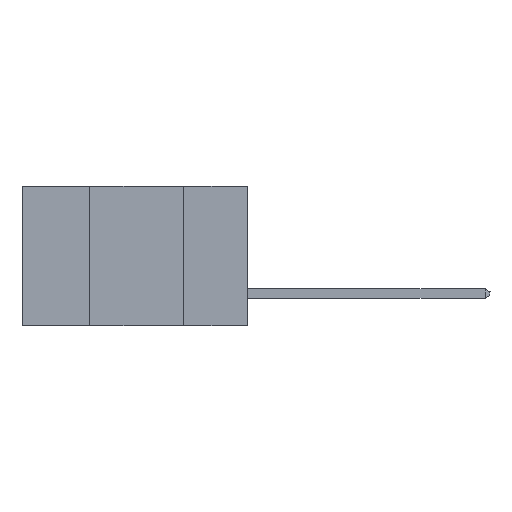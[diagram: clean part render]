
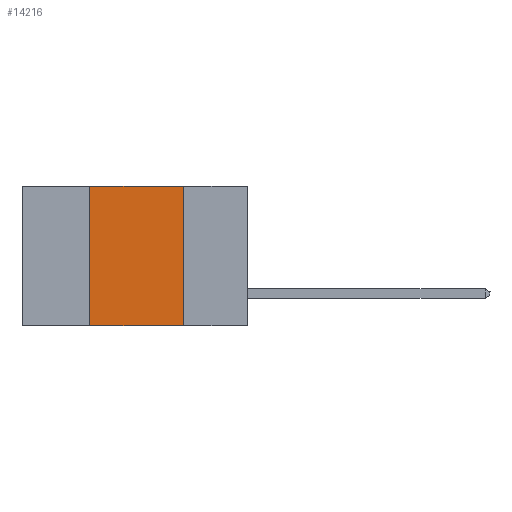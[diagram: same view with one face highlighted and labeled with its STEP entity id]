
A CAD part, left-side view. The second image highlights one B-rep face of the part: STEP entity #14216.
In plain terms, the highlighted planar face has unit normal (-1, 0, 0).
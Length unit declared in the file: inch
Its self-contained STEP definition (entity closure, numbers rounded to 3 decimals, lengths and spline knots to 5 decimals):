
#107 = CARTESIAN_POINT ( 'NONE',  ( 0., 0.17, -0.37 ) ) ;
#370 = VECTOR ( 'NONE', #12506, 39.37008 ) ;
#591 = LINE ( 'NONE', #22210, #370 ) ;
#2388 = LINE ( 'NONE', #23874, #9001 ) ;
#3437 = DIRECTION ( 'NONE',  ( 1., 0., 0. ) ) ;
#3666 = ORIENTED_EDGE ( 'NONE', *, *, #16889, .F. ) ;
#3943 = LINE ( 'NONE', #25311, #14089 ) ;
#4243 = CARTESIAN_POINT ( 'NONE',  ( 0., 0.42, -0.37 ) ) ;
#4478 = AXIS2_PLACEMENT_3D ( 'NONE', #17686, #3437, #25567 ) ;
#5804 = EDGE_CURVE ( 'NONE', #6952, #15872, #2388, .T. ) ;
#6952 = VERTEX_POINT ( 'NONE', #22259 ) ;
#7574 = LINE ( 'NONE', #17552, #21481 ) ;
#9001 = VECTOR ( 'NONE', #10285, 39.37008 ) ;
#10285 = DIRECTION ( 'NONE',  ( 0., -1., 0. ) ) ;
#10796 = CARTESIAN_POINT ( 'NONE',  ( 0., 0.17, 0. ) ) ;
#10942 = FACE_OUTER_BOUND ( 'NONE', #14333, .T. ) ;
#12285 = ORIENTED_EDGE ( 'NONE', *, *, #12989, .T. ) ;
#12506 = DIRECTION ( 'NONE',  ( 0., 0., 1. ) ) ;
#12700 = EDGE_CURVE ( 'NONE', #21989, #6952, #591, .T. ) ;
#12989 = EDGE_CURVE ( 'NONE', #21989, #23261, #7574, .T. ) ;
#14089 = VECTOR ( 'NONE', #23353, 39.37008 ) ;
#14216 = ADVANCED_FACE ( 'NONE', ( #10942 ), #18850, .F. ) ;
#14333 = EDGE_LOOP ( 'NONE', ( #3666, #20931, #16281, #12285 ) ) ;
#15872 = VERTEX_POINT ( 'NONE', #10796 ) ;
#16281 = ORIENTED_EDGE ( 'NONE', *, *, #12700, .F. ) ;
#16889 = EDGE_CURVE ( 'NONE', #15872, #23261, #3943, .T. ) ;
#17552 = CARTESIAN_POINT ( 'NONE',  ( 0., 0.6, -0.37 ) ) ;
#17686 = CARTESIAN_POINT ( 'NONE',  ( 0., 0.6, 0. ) ) ;
#18850 = PLANE ( 'NONE',  #4478 ) ;
#20931 = ORIENTED_EDGE ( 'NONE', *, *, #5804, .F. ) ;
#21481 = VECTOR ( 'NONE', #23613, 39.37008 ) ;
#21989 = VERTEX_POINT ( 'NONE', #4243 ) ;
#22210 = CARTESIAN_POINT ( 'NONE',  ( 0., 0.42, -0.37 ) ) ;
#22259 = CARTESIAN_POINT ( 'NONE',  ( 0., 0.42, 0. ) ) ;
#23261 = VERTEX_POINT ( 'NONE', #107 ) ;
#23353 = DIRECTION ( 'NONE',  ( 0., 0., -1. ) ) ;
#23613 = DIRECTION ( 'NONE',  ( 0., -1., 0. ) ) ;
#23874 = CARTESIAN_POINT ( 'NONE',  ( 0., 0.6, 0. ) ) ;
#25311 = CARTESIAN_POINT ( 'NONE',  ( 0., 0.17, -0.37 ) ) ;
#25567 = DIRECTION ( 'NONE',  ( 0., 0., -1. ) ) ;
